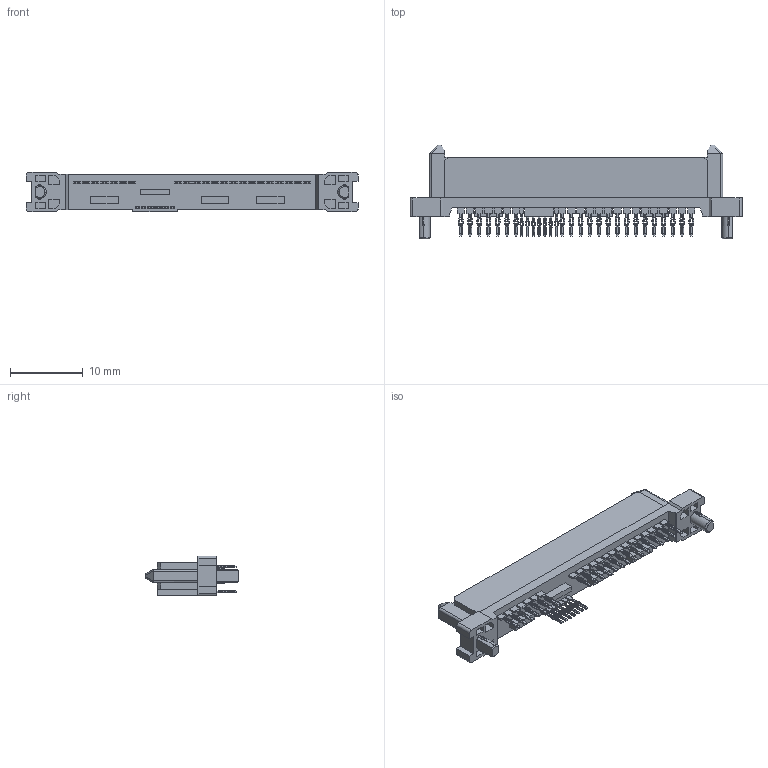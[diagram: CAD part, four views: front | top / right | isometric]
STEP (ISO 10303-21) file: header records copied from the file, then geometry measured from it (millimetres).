
FILE_DESCRIPTION (( 'STEP AP214' ), '1' );
FILE_NAME ('272-029-631-002.STEP', '2020-05-19T13:04:43', ( '' ), ( '' ), 'SwSTEP 2.0', 'SolidWorks 2020', '' );
FILE_SCHEMA (( 'AUTOMOTIVE_DESIGN' ));
Length unit declared in the file: centimetre
Products named in the file (3): 272-029-631-002; 272-029-631-002 Body; 272-029-631-002 tail
Assembly tree (2 placements, depth 2):
  272-029-631-002
    272-029-631-002 Body
    272-029-631-002 tail
Bounding box: 45.75 x 12.95 x 5.5 mm (x, y, z)
Volume: 923.9 mm3; surface area: 1953.4 mm2
Topology: 30 solids, 30 shells, 2525 faces, 6606 edges, 4166 vertices
Faces by surface type: cylinder 1078, plane 978, bspline 464, cone 5
Entity records: 111697 total; most frequent: CARTESIAN_POINT 25580, ORIENTED_EDGE 13212, DIRECTION 11080, EDGE_CURVE 6606, VERTEX_POINT 4166, AXIS2_PLACEMENT_3D 3728, LINE 3624, VECTOR 3624
